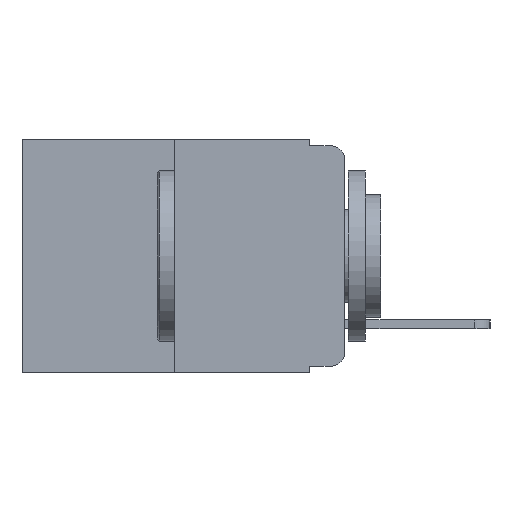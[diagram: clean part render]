
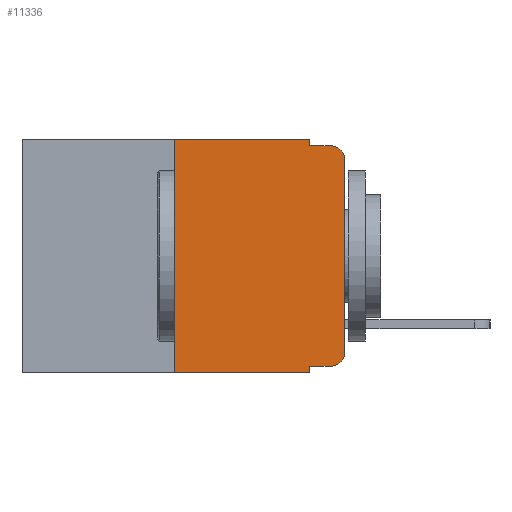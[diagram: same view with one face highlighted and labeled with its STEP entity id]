
A CAD part, left-side view. The second image highlights one B-rep face of the part: STEP entity #11336.
In plain terms, the highlighted planar face has unit normal (-1, 0, 0).
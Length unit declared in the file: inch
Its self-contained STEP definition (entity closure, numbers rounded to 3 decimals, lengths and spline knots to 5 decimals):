
#295 = LINE ( 'NONE', #6824, #8470 ) ;
#1138 = LINE ( 'NONE', #7091, #12269 ) ;
#1246 = VECTOR ( 'NONE', #10867, 39.37008 ) ;
#1977 = VECTOR ( 'NONE', #17584, 39.37008 ) ;
#2635 = AXIS2_PLACEMENT_3D ( 'NONE', #5682, #4063, #18792 ) ;
#2678 = VERTEX_POINT ( 'NONE', #14113 ) ;
#3002 = VERTEX_POINT ( 'NONE', #10555 ) ;
#3016 = DIRECTION ( 'NONE',  ( 0., -1., 0. ) ) ;
#3025 = VERTEX_POINT ( 'NONE', #3222 ) ;
#3181 = DIRECTION ( 'NONE',  ( -1., 0., 0. ) ) ;
#3222 = CARTESIAN_POINT ( 'NONE',  ( 0., 0.25, -0.343 ) ) ;
#3322 = CARTESIAN_POINT ( 'NONE',  ( 0., 0.25, 0. ) ) ;
#3408 = CARTESIAN_POINT ( 'NONE',  ( 0., 0.02, -0.333 ) ) ;
#3815 = EDGE_CURVE ( 'NONE', #3025, #7131, #5621, .T. ) ;
#3943 = CARTESIAN_POINT ( 'NONE',  ( 0., 0.25, 0. ) ) ;
#4011 = VECTOR ( 'NONE', #5895, 39.37008 ) ;
#4063 = DIRECTION ( 'NONE',  ( 1., 0., 0. ) ) ;
#4345 = VECTOR ( 'NONE', #15585, 39.37008 ) ;
#4577 = DIRECTION ( 'NONE',  ( -1., 0., 0. ) ) ;
#5222 = CARTESIAN_POINT ( 'NONE',  ( 0., 0.473, 0. ) ) ;
#5372 = LINE ( 'NONE', #16655, #1246 ) ;
#5556 = DIRECTION ( 'NONE',  ( 0., -1., 0. ) ) ;
#5621 = LINE ( 'NONE', #3322, #16893 ) ;
#5682 = CARTESIAN_POINT ( 'NONE',  ( 0., 0.473, 0. ) ) ;
#5864 = VERTEX_POINT ( 'NONE', #15104 ) ;
#5895 = DIRECTION ( 'NONE',  ( 0., 0., -1. ) ) ;
#6389 = EDGE_CURVE ( 'NONE', #8893, #7715, #13981, .T. ) ;
#6824 = CARTESIAN_POINT ( 'NONE',  ( 0., 0., 0. ) ) ;
#7032 = ORIENTED_EDGE ( 'NONE', *, *, #15916, .T. ) ;
#7091 = CARTESIAN_POINT ( 'NONE',  ( 0., 0.051, -0.01 ) ) ;
#7131 = VERTEX_POINT ( 'NONE', #3943 ) ;
#7394 = CARTESIAN_POINT ( 'NONE',  ( 0., 0.051, 0. ) ) ;
#7715 = VERTEX_POINT ( 'NONE', #14502 ) ;
#7984 = VERTEX_POINT ( 'NONE', #16564 ) ;
#8157 = AXIS2_PLACEMENT_3D ( 'NONE', #12204, #3181, #13662 ) ;
#8417 = ORIENTED_EDGE ( 'NONE', *, *, #11995, .T. ) ;
#8470 = VECTOR ( 'NONE', #15638, 39.37008 ) ;
#8515 = LINE ( 'NONE', #13341, #4011 ) ;
#8893 = VERTEX_POINT ( 'NONE', #13194 ) ;
#9104 = EDGE_CURVE ( 'NONE', #10271, #7984, #18099, .T. ) ;
#9297 = LINE ( 'NONE', #5222, #4345 ) ;
#9336 = ORIENTED_EDGE ( 'NONE', *, *, #14324, .T. ) ;
#9833 = ORIENTED_EDGE ( 'NONE', *, *, #14600, .F. ) ;
#10271 = VERTEX_POINT ( 'NONE', #3408 ) ;
#10378 = EDGE_LOOP ( 'NONE', ( #18168, #7032, #15779, #12885, #9833, #17521, #8417, #12868, #9336, #13309 ) ) ;
#10552 = FACE_OUTER_BOUND ( 'NONE', #10378, .T. ) ;
#10555 = CARTESIAN_POINT ( 'NONE',  ( 0., 0.051, -0.333 ) ) ;
#10788 = AXIS2_PLACEMENT_3D ( 'NONE', #13538, #4577, #14987 ) ;
#10867 = DIRECTION ( 'NONE',  ( 0., -1., 0. ) ) ;
#10902 = CIRCLE ( 'NONE', #10788, 0.02 ) ;
#11204 = EDGE_CURVE ( 'NONE', #7984, #2678, #295, .T. ) ;
#11336 = ADVANCED_FACE ( 'NONE', ( #10552 ), #17397, .F. ) ;
#11468 = VERTEX_POINT ( 'NONE', #17689 ) ;
#11995 = EDGE_CURVE ( 'NONE', #3025, #11468, #5372, .T. ) ;
#12204 = CARTESIAN_POINT ( 'NONE',  ( 0., 0.02, -0.313 ) ) ;
#12269 = VECTOR ( 'NONE', #5556, 39.37008 ) ;
#12352 = DIRECTION ( 'NONE',  ( 0., 0., 1. ) ) ;
#12868 = ORIENTED_EDGE ( 'NONE', *, *, #18680, .F. ) ;
#12885 = ORIENTED_EDGE ( 'NONE', *, *, #6389, .F. ) ;
#13194 = CARTESIAN_POINT ( 'NONE',  ( 0., 0.051, 0. ) ) ;
#13309 = ORIENTED_EDGE ( 'NONE', *, *, #9104, .T. ) ;
#13341 = CARTESIAN_POINT ( 'NONE',  ( 0., 0.051, 0. ) ) ;
#13453 = CARTESIAN_POINT ( 'NONE',  ( 0., 0.051, -0.333 ) ) ;
#13538 = CARTESIAN_POINT ( 'NONE',  ( 0., 0.02, -0.03 ) ) ;
#13662 = DIRECTION ( 'NONE',  ( 0., 0., -1. ) ) ;
#13945 = LINE ( 'NONE', #13453, #17278 ) ;
#13981 = LINE ( 'NONE', #7394, #1977 ) ;
#14113 = CARTESIAN_POINT ( 'NONE',  ( 0., 0., -0.03 ) ) ;
#14324 = EDGE_CURVE ( 'NONE', #3002, #10271, #13945, .T. ) ;
#14502 = CARTESIAN_POINT ( 'NONE',  ( 0., 0.051, -0.01 ) ) ;
#14600 = EDGE_CURVE ( 'NONE', #7131, #8893, #9297, .T. ) ;
#14987 = DIRECTION ( 'NONE',  ( 0., 0., -1. ) ) ;
#15104 = CARTESIAN_POINT ( 'NONE',  ( 0., 0.02, -0.01 ) ) ;
#15585 = DIRECTION ( 'NONE',  ( 0., -1., 0. ) ) ;
#15638 = DIRECTION ( 'NONE',  ( 0., 0., 1. ) ) ;
#15779 = ORIENTED_EDGE ( 'NONE', *, *, #16849, .F. ) ;
#15916 = EDGE_CURVE ( 'NONE', #2678, #5864, #10902, .T. ) ;
#16564 = CARTESIAN_POINT ( 'NONE',  ( 0., 0., -0.313 ) ) ;
#16655 = CARTESIAN_POINT ( 'NONE',  ( 0., 0.473, -0.343 ) ) ;
#16849 = EDGE_CURVE ( 'NONE', #7715, #5864, #1138, .T. ) ;
#16893 = VECTOR ( 'NONE', #12352, 39.37008 ) ;
#17278 = VECTOR ( 'NONE', #3016, 39.37008 ) ;
#17397 = PLANE ( 'NONE',  #2635 ) ;
#17521 = ORIENTED_EDGE ( 'NONE', *, *, #3815, .F. ) ;
#17584 = DIRECTION ( 'NONE',  ( 0., 0., -1. ) ) ;
#17689 = CARTESIAN_POINT ( 'NONE',  ( 0., 0.051, -0.343 ) ) ;
#18099 = CIRCLE ( 'NONE', #8157, 0.02 ) ;
#18168 = ORIENTED_EDGE ( 'NONE', *, *, #11204, .T. ) ;
#18680 = EDGE_CURVE ( 'NONE', #3002, #11468, #8515, .T. ) ;
#18792 = DIRECTION ( 'NONE',  ( 0., 0., -1. ) ) ;
